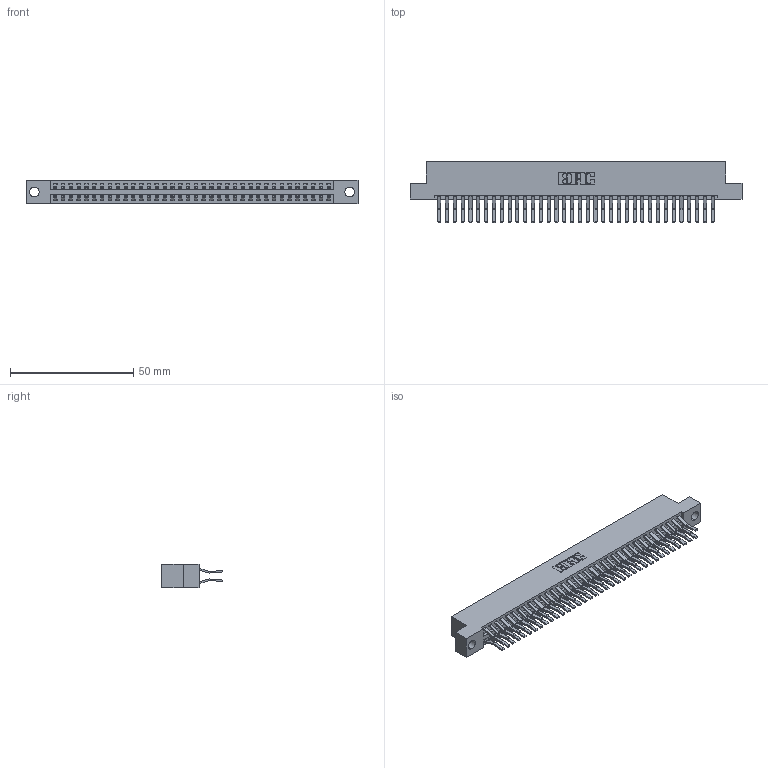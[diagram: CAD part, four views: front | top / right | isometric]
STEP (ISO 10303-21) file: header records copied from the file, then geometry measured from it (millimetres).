
FILE_DESCRIPTION (( 'STEP AP203' ), '1' );
FILE_NAME ('346-072-560-204.STEP', '2022-05-25T01:11:46', ( '' ), ( '' ), 'SwSTEP 2.0', 'SolidWorks 2020', '' );
FILE_SCHEMA (( 'CONFIG_CONTROL_DESIGN' ));
Length unit declared in the file: inch
Products named in the file (3): 345-292-001_560 Tail; 346-072-560-204; 346 Part_Flush Mounting Lugs - 0.156 Dia-TH
Assembly tree (73 placements, depth 2):
  346-072-560-204
    346 Part_Flush Mounting Lugs - 0.156 Dia-TH
    345-292-001_560 Tail  x72
Bounding box: 134.87 x 24.78 x 9.4 mm (x, y, z)
Volume: 13471.3 mm3; surface area: 19529.8 mm2
Topology: 73 solids, 73 shells, 4024 faces, 11957 edges, 7874 vertices
Faces by surface type: plane 2610, cylinder 1414
Entity records: 24809 total; most frequent: CARTESIAN_POINT 4102, ORIENTED_EDGE 4034, DIRECTION 3669, EDGE_CURVE 2017, VECTOR 1737, LINE 1737, VERTEX_POINT 1342, AXIS2_PLACEMENT_3D 966
